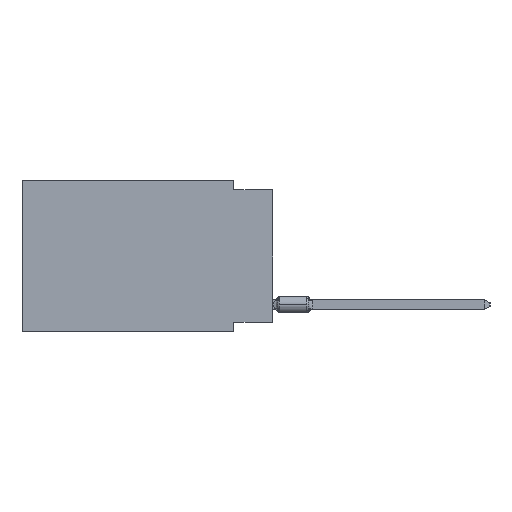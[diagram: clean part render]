
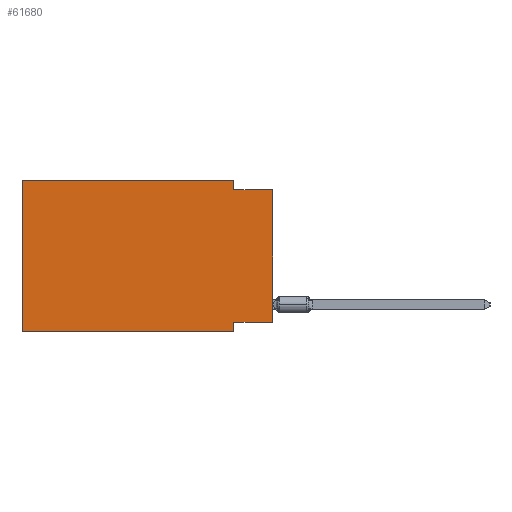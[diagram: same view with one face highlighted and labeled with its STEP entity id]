
A CAD part, left-side view. The second image highlights one B-rep face of the part: STEP entity #61680.
In plain terms, the highlighted planar face has unit normal (-1, 0, 0).
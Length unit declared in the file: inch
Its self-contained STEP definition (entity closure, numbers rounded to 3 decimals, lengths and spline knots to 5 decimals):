
#501 = LINE ( 'NONE', #60804, #29200 ) ;
#1758 = CARTESIAN_POINT ( 'NONE',  ( 0., 0., -0.365 ) ) ;
#1863 = VECTOR ( 'NONE', #37699, 39.37008 ) ;
#2184 = VERTEX_POINT ( 'NONE', #8184 ) ;
#2270 = EDGE_CURVE ( 'NONE', #2184, #43279, #27168, .T. ) ;
#2296 = DIRECTION ( 'NONE',  ( 0., 0., -1. ) ) ;
#4581 = ORIENTED_EDGE ( 'NONE', *, *, #20116, .F. ) ;
#6665 = DIRECTION ( 'NONE',  ( 0., 0., -1. ) ) ;
#6794 = LINE ( 'NONE', #61890, #54991 ) ;
#8184 = CARTESIAN_POINT ( 'NONE',  ( 0., 0.1, 0. ) ) ;
#8323 = CARTESIAN_POINT ( 'NONE',  ( 0., 0.1, -0.025 ) ) ;
#9071 = LINE ( 'NONE', #15591, #32082 ) ;
#11926 = VERTEX_POINT ( 'NONE', #14574 ) ;
#12162 = EDGE_CURVE ( 'NONE', #43279, #11926, #501, .T. ) ;
#13120 = DIRECTION ( 'NONE',  ( 0., 0., 1. ) ) ;
#13957 = CARTESIAN_POINT ( 'NONE',  ( 0., 0.645, 0. ) ) ;
#14574 = CARTESIAN_POINT ( 'NONE',  ( 0., 0., -0.025 ) ) ;
#15133 = VECTOR ( 'NONE', #6665, 39.37008 ) ;
#15591 = CARTESIAN_POINT ( 'NONE',  ( 0., 0.645, -0.39 ) ) ;
#16273 = CARTESIAN_POINT ( 'NONE',  ( 0., 0.645, 0. ) ) ;
#17173 = VERTEX_POINT ( 'NONE', #45206 ) ;
#17260 = EDGE_LOOP ( 'NONE', ( #62093, #31101, #58367, #27038, #55386, #62012, #4581, #64350 ) ) ;
#17751 = VERTEX_POINT ( 'NONE', #23003 ) ;
#18212 = DIRECTION ( 'NONE',  ( 0., 0., 1. ) ) ;
#19494 = DIRECTION ( 'NONE',  ( 0., 0., -1. ) ) ;
#20116 = EDGE_CURVE ( 'NONE', #17751, #17173, #21722, .T. ) ;
#21331 = VERTEX_POINT ( 'NONE', #1758 ) ;
#21718 = EDGE_CURVE ( 'NONE', #21331, #17751, #47864, .T. ) ;
#21722 = LINE ( 'NONE', #35840, #15133 ) ;
#22495 = VERTEX_POINT ( 'NONE', #16273 ) ;
#23003 = CARTESIAN_POINT ( 'NONE',  ( 0., 0.1, -0.365 ) ) ;
#23756 = PLANE ( 'NONE',  #31260 ) ;
#26519 = EDGE_CURVE ( 'NONE', #21331, #11926, #58039, .T. ) ;
#27038 = ORIENTED_EDGE ( 'NONE', *, *, #31643, .F. ) ;
#27168 = LINE ( 'NONE', #58020, #63383 ) ;
#28697 = LINE ( 'NONE', #13957, #48844 ) ;
#29200 = VECTOR ( 'NONE', #42373, 39.37008 ) ;
#29782 = CARTESIAN_POINT ( 'NONE',  ( 0., 0.645, -0.39 ) ) ;
#31101 = ORIENTED_EDGE ( 'NONE', *, *, #12162, .F. ) ;
#31260 = AXIS2_PLACEMENT_3D ( 'NONE', #39484, #34238, #19494 ) ;
#31643 = EDGE_CURVE ( 'NONE', #22495, #2184, #6794, .T. ) ;
#32082 = VECTOR ( 'NONE', #60210, 39.37008 ) ;
#33265 = FACE_OUTER_BOUND ( 'NONE', #17260, .T. ) ;
#34238 = DIRECTION ( 'NONE',  ( 1., 0., 0. ) ) ;
#35840 = CARTESIAN_POINT ( 'NONE',  ( 0., 0.1, -0.39 ) ) ;
#37699 = DIRECTION ( 'NONE',  ( 0., 1., 0. ) ) ;
#37868 = VECTOR ( 'NONE', #13120, 39.37008 ) ;
#39484 = CARTESIAN_POINT ( 'NONE',  ( 0., 0.645, 0. ) ) ;
#42373 = DIRECTION ( 'NONE',  ( 0., -1., 0. ) ) ;
#43266 = CARTESIAN_POINT ( 'NONE',  ( 0., 0., 0. ) ) ;
#43279 = VERTEX_POINT ( 'NONE', #8323 ) ;
#45206 = CARTESIAN_POINT ( 'NONE',  ( 0., 0.1, -0.39 ) ) ;
#45443 = VERTEX_POINT ( 'NONE', #29782 ) ;
#47293 = EDGE_CURVE ( 'NONE', #45443, #22495, #28697, .T. ) ;
#47864 = LINE ( 'NONE', #62331, #1863 ) ;
#48844 = VECTOR ( 'NONE', #18212, 39.37008 ) ;
#54991 = VECTOR ( 'NONE', #56329, 39.37008 ) ;
#55386 = ORIENTED_EDGE ( 'NONE', *, *, #47293, .F. ) ;
#56329 = DIRECTION ( 'NONE',  ( 0., -1., 0. ) ) ;
#58020 = CARTESIAN_POINT ( 'NONE',  ( 0., 0.1, 0. ) ) ;
#58039 = LINE ( 'NONE', #43266, #37868 ) ;
#58367 = ORIENTED_EDGE ( 'NONE', *, *, #2270, .F. ) ;
#60210 = DIRECTION ( 'NONE',  ( 0., -1., 0. ) ) ;
#60774 = EDGE_CURVE ( 'NONE', #45443, #17173, #9071, .T. ) ;
#60804 = CARTESIAN_POINT ( 'NONE',  ( 0., 0., -0.025 ) ) ;
#61680 = ADVANCED_FACE ( 'NONE', ( #33265 ), #23756, .F. ) ;
#61890 = CARTESIAN_POINT ( 'NONE',  ( 0., 0.645, 0. ) ) ;
#62012 = ORIENTED_EDGE ( 'NONE', *, *, #60774, .T. ) ;
#62093 = ORIENTED_EDGE ( 'NONE', *, *, #26519, .T. ) ;
#62331 = CARTESIAN_POINT ( 'NONE',  ( 0., 0., -0.365 ) ) ;
#63383 = VECTOR ( 'NONE', #2296, 39.37008 ) ;
#64350 = ORIENTED_EDGE ( 'NONE', *, *, #21718, .F. ) ;
